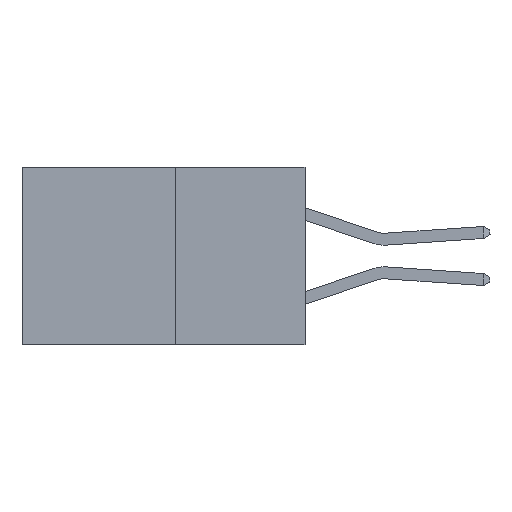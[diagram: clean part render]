
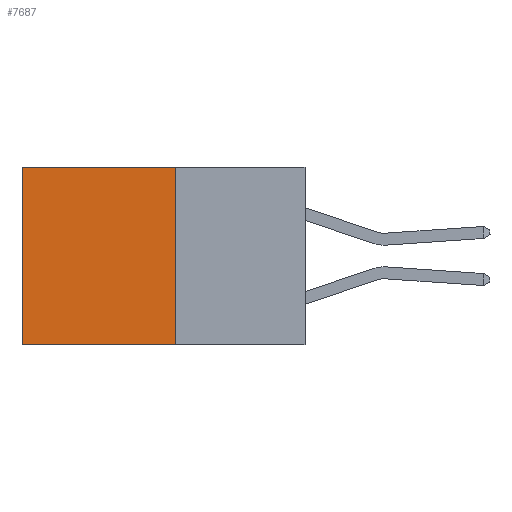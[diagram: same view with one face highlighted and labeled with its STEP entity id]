
A CAD part, left-side view. The second image highlights one B-rep face of the part: STEP entity #7687.
In plain terms, the highlighted planar face has unit normal (-1, 0, 0).
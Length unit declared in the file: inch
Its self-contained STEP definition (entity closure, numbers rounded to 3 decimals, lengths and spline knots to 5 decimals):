
#1245 = VECTOR ( 'NONE', #11450, 39.37008 ) ;
#1843 = LINE ( 'NONE', #6290, #5051 ) ;
#3314 = VERTEX_POINT ( 'NONE', #11800 ) ;
#3494 = ORIENTED_EDGE ( 'NONE', *, *, #9992, .T. ) ;
#3618 = VERTEX_POINT ( 'NONE', #15729 ) ;
#3717 = ORIENTED_EDGE ( 'NONE', *, *, #4412, .F. ) ;
#3750 = ORIENTED_EDGE ( 'NONE', *, *, #4043, .F. ) ;
#4043 = EDGE_CURVE ( 'NONE', #3314, #3618, #1843, .T. ) ;
#4370 = ORIENTED_EDGE ( 'NONE', *, *, #8915, .T. ) ;
#4412 = EDGE_CURVE ( 'NONE', #3618, #13441, #5766, .T. ) ;
#5051 = VECTOR ( 'NONE', #6107, 39.37008 ) ;
#5766 = LINE ( 'NONE', #16156, #12416 ) ;
#6107 = DIRECTION ( 'NONE',  ( 0., 0., -1. ) ) ;
#6277 = FACE_OUTER_BOUND ( 'NONE', #13471, .T. ) ;
#6290 = CARTESIAN_POINT ( 'NONE',  ( 0.277, 0.27, -0.37 ) ) ;
#7050 = CARTESIAN_POINT ( 'NONE',  ( 0.277, 0.27, -0.37 ) ) ;
#7687 = ADVANCED_FACE ( 'NONE', ( #6277 ), #14453, .F. ) ;
#8149 = LINE ( 'NONE', #10189, #1245 ) ;
#8309 = DIRECTION ( 'NONE',  ( 0., 0., -1. ) ) ;
#8915 = EDGE_CURVE ( 'NONE', #3314, #12713, #15823, .T. ) ;
#9992 = EDGE_CURVE ( 'NONE', #12713, #13441, #8149, .T. ) ;
#10189 = CARTESIAN_POINT ( 'NONE',  ( 0.277, 0.59, -0.37 ) ) ;
#11018 = CARTESIAN_POINT ( 'NONE',  ( 0.277, 0.59, -0.37 ) ) ;
#11450 = DIRECTION ( 'NONE',  ( 0., 0., -1. ) ) ;
#11800 = CARTESIAN_POINT ( 'NONE',  ( 0.277, 0.27, 0. ) ) ;
#12416 = VECTOR ( 'NONE', #15995, 39.37008 ) ;
#12695 = VECTOR ( 'NONE', #15605, 39.37008 ) ;
#12713 = VERTEX_POINT ( 'NONE', #15921 ) ;
#13441 = VERTEX_POINT ( 'NONE', #11018 ) ;
#13471 = EDGE_LOOP ( 'NONE', ( #3494, #3717, #3750, #4370 ) ) ;
#14142 = AXIS2_PLACEMENT_3D ( 'NONE', #7050, #15646, #8309 ) ;
#14412 = CARTESIAN_POINT ( 'NONE',  ( 0.277, 0.27, 0. ) ) ;
#14453 = PLANE ( 'NONE',  #14142 ) ;
#15605 = DIRECTION ( 'NONE',  ( 0., 1., 0. ) ) ;
#15646 = DIRECTION ( 'NONE',  ( 1., 0., 0. ) ) ;
#15729 = CARTESIAN_POINT ( 'NONE',  ( 0.277, 0.27, -0.37 ) ) ;
#15823 = LINE ( 'NONE', #14412, #12695 ) ;
#15921 = CARTESIAN_POINT ( 'NONE',  ( 0.277, 0.59, 0. ) ) ;
#15995 = DIRECTION ( 'NONE',  ( 0., 1., 0. ) ) ;
#16156 = CARTESIAN_POINT ( 'NONE',  ( 0.277, 0.27, -0.37 ) ) ;
